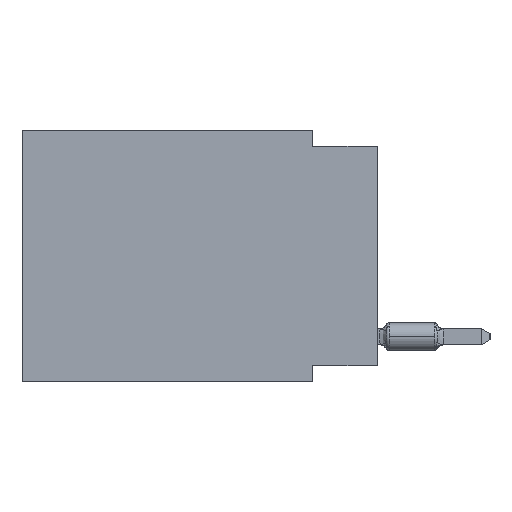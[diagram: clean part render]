
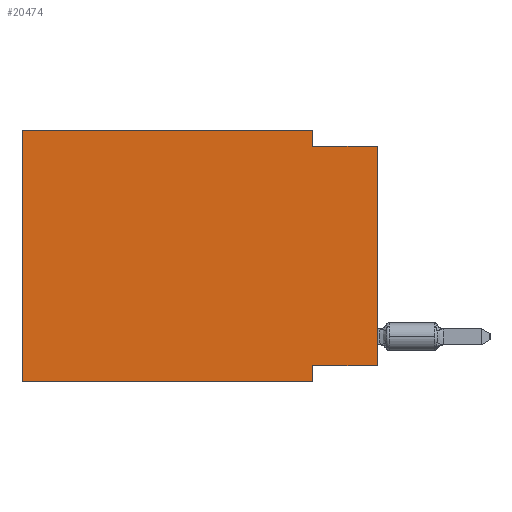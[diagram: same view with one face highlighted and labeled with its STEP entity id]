
A CAD part, left-side view. The second image highlights one B-rep face of the part: STEP entity #20474.
In plain terms, the highlighted planar face has unit normal (-1, 0, 0).
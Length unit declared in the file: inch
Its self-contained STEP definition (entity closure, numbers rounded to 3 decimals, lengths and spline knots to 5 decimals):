
#1455 = CARTESIAN_POINT ( 'NONE',  ( 0., 0.1, -0.39 ) ) ;
#1961 = LINE ( 'NONE', #20277, #9802 ) ;
#3643 = CARTESIAN_POINT ( 'NONE',  ( 0., 0.1, -0.365 ) ) ;
#3721 = ORIENTED_EDGE ( 'NONE', *, *, #6270, .F. ) ;
#4255 = CARTESIAN_POINT ( 'NONE',  ( 0., 0.1, -0.025 ) ) ;
#5278 = VECTOR ( 'NONE', #29597, 39.37008 ) ;
#6093 = ORIENTED_EDGE ( 'NONE', *, *, #12855, .T. ) ;
#6270 = EDGE_CURVE ( 'NONE', #11813, #23239, #25795, .T. ) ;
#7937 = VERTEX_POINT ( 'NONE', #24596 ) ;
#8628 = LINE ( 'NONE', #22187, #35594 ) ;
#9343 = DIRECTION ( 'NONE',  ( 0., 0., -1. ) ) ;
#9802 = VECTOR ( 'NONE', #9343, 39.37008 ) ;
#10177 = CARTESIAN_POINT ( 'NONE',  ( 0., 0.55, 0. ) ) ;
#11813 = VERTEX_POINT ( 'NONE', #4255 ) ;
#12855 = EDGE_CURVE ( 'NONE', #22096, #23239, #32937, .T. ) ;
#12971 = VERTEX_POINT ( 'NONE', #15818 ) ;
#14395 = CARTESIAN_POINT ( 'NONE',  ( 0., 0., 0. ) ) ;
#14471 = CARTESIAN_POINT ( 'NONE',  ( 0., 0.55, 0. ) ) ;
#14874 = DIRECTION ( 'NONE',  ( 0., 0., 1. ) ) ;
#15818 = CARTESIAN_POINT ( 'NONE',  ( 0., 0.1, 0. ) ) ;
#16173 = CARTESIAN_POINT ( 'NONE',  ( 0., 0.55, -0.39 ) ) ;
#16329 = CARTESIAN_POINT ( 'NONE',  ( 0., 0.55, 0. ) ) ;
#16830 = EDGE_CURVE ( 'NONE', #32847, #7937, #38779, .T. ) ;
#16898 = ORIENTED_EDGE ( 'NONE', *, *, #30866, .F. ) ;
#17029 = VECTOR ( 'NONE', #14874, 39.37008 ) ;
#17074 = EDGE_CURVE ( 'NONE', #23811, #43544, #26781, .T. ) ;
#18280 = DIRECTION ( 'NONE',  ( 0., -1., 0. ) ) ;
#18614 = DIRECTION ( 'NONE',  ( 0., 1., 0. ) ) ;
#18861 = EDGE_LOOP ( 'NONE', ( #6093, #3721, #21681, #16898, #46501, #25419, #21958, #26563 ) ) ;
#19715 = VECTOR ( 'NONE', #41148, 39.37008 ) ;
#20277 = CARTESIAN_POINT ( 'NONE',  ( 0., 0.1, 0. ) ) ;
#20474 = ADVANCED_FACE ( 'NONE', ( #46553 ), #39889, .F. ) ;
#21681 = ORIENTED_EDGE ( 'NONE', *, *, #42536, .F. ) ;
#21958 = ORIENTED_EDGE ( 'NONE', *, *, #16830, .F. ) ;
#22001 = CARTESIAN_POINT ( 'NONE',  ( 0., 0., -0.365 ) ) ;
#22096 = VERTEX_POINT ( 'NONE', #22001 ) ;
#22187 = CARTESIAN_POINT ( 'NONE',  ( 0., 0., -0.365 ) ) ;
#23223 = EDGE_CURVE ( 'NONE', #23811, #7937, #24009, .T. ) ;
#23239 = VERTEX_POINT ( 'NONE', #30428 ) ;
#23811 = VERTEX_POINT ( 'NONE', #31320 ) ;
#24009 = LINE ( 'NONE', #16173, #19715 ) ;
#24596 = CARTESIAN_POINT ( 'NONE',  ( 0., 0.1, -0.39 ) ) ;
#25419 = ORIENTED_EDGE ( 'NONE', *, *, #23223, .T. ) ;
#25795 = LINE ( 'NONE', #29128, #5278 ) ;
#26563 = ORIENTED_EDGE ( 'NONE', *, *, #42448, .F. ) ;
#26781 = LINE ( 'NONE', #16329, #42962 ) ;
#29128 = CARTESIAN_POINT ( 'NONE',  ( 0., 0., -0.025 ) ) ;
#29597 = DIRECTION ( 'NONE',  ( 0., -1., 0. ) ) ;
#30428 = CARTESIAN_POINT ( 'NONE',  ( 0., 0., -0.025 ) ) ;
#30866 = EDGE_CURVE ( 'NONE', #43544, #12971, #47059, .T. ) ;
#31320 = CARTESIAN_POINT ( 'NONE',  ( 0., 0.55, -0.39 ) ) ;
#31811 = DIRECTION ( 'NONE',  ( 0., 0., -1. ) ) ;
#32762 = VECTOR ( 'NONE', #18280, 39.37008 ) ;
#32847 = VERTEX_POINT ( 'NONE', #3643 ) ;
#32937 = LINE ( 'NONE', #14395, #17029 ) ;
#33179 = AXIS2_PLACEMENT_3D ( 'NONE', #10177, #40124, #31811 ) ;
#33853 = CARTESIAN_POINT ( 'NONE',  ( 0., 0.55, 0. ) ) ;
#34175 = DIRECTION ( 'NONE',  ( 0., 0., 1. ) ) ;
#34993 = DIRECTION ( 'NONE',  ( 0., 0., -1. ) ) ;
#35594 = VECTOR ( 'NONE', #18614, 39.37008 ) ;
#37652 = VECTOR ( 'NONE', #34993, 39.37008 ) ;
#38779 = LINE ( 'NONE', #1455, #37652 ) ;
#39889 = PLANE ( 'NONE',  #33179 ) ;
#40124 = DIRECTION ( 'NONE',  ( 1., 0., 0. ) ) ;
#41148 = DIRECTION ( 'NONE',  ( 0., -1., 0. ) ) ;
#42448 = EDGE_CURVE ( 'NONE', #22096, #32847, #8628, .T. ) ;
#42536 = EDGE_CURVE ( 'NONE', #12971, #11813, #1961, .T. ) ;
#42962 = VECTOR ( 'NONE', #34175, 39.37008 ) ;
#43544 = VERTEX_POINT ( 'NONE', #33853 ) ;
#46501 = ORIENTED_EDGE ( 'NONE', *, *, #17074, .F. ) ;
#46553 = FACE_OUTER_BOUND ( 'NONE', #18861, .T. ) ;
#47059 = LINE ( 'NONE', #14471, #32762 ) ;
